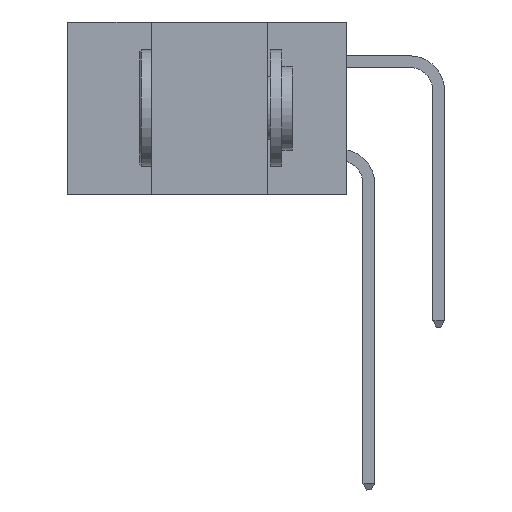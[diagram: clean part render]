
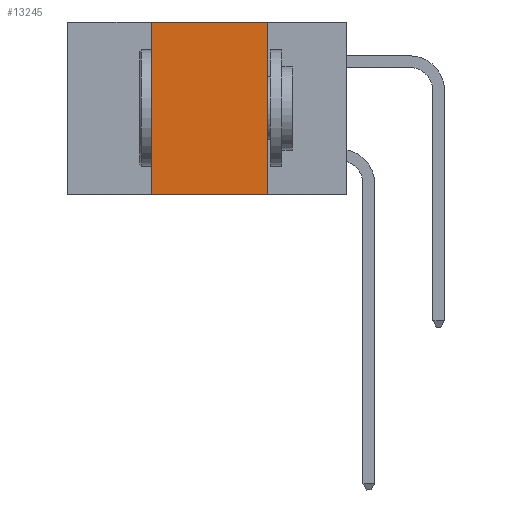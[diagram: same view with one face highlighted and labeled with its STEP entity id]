
A CAD part, left-side view. The second image highlights one B-rep face of the part: STEP entity #13245.
In plain terms, the highlighted planar face has unit normal (-1, 0, 0).
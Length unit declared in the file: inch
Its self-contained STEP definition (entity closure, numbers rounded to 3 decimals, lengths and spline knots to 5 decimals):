
#2314 = CARTESIAN_POINT ( 'NONE',  ( 0., 0.6, 0. ) ) ;
#2728 = VECTOR ( 'NONE', #20576, 39.37008 ) ;
#3229 = VERTEX_POINT ( 'NONE', #11223 ) ;
#3292 = EDGE_CURVE ( 'NONE', #20865, #9511, #11533, .T. ) ;
#3324 = EDGE_CURVE ( 'NONE', #19176, #20865, #10949, .T. ) ;
#3761 = CARTESIAN_POINT ( 'NONE',  ( 0., 0.42, 0. ) ) ;
#4230 = PLANE ( 'NONE',  #18257 ) ;
#5069 = DIRECTION ( 'NONE',  ( 0., 0., -1. ) ) ;
#7204 = VECTOR ( 'NONE', #10216, 39.37008 ) ;
#7755 = LINE ( 'NONE', #9397, #2728 ) ;
#7993 = DIRECTION ( 'NONE',  ( 1., 0., 0. ) ) ;
#9397 = CARTESIAN_POINT ( 'NONE',  ( 0., 0.6, -0.37 ) ) ;
#9511 = VERTEX_POINT ( 'NONE', #19887 ) ;
#9880 = CARTESIAN_POINT ( 'NONE',  ( 0., 0.42, 0. ) ) ;
#10057 = DIRECTION ( 'NONE',  ( 0., 0., 1. ) ) ;
#10216 = DIRECTION ( 'NONE',  ( 0., -1., 0. ) ) ;
#10287 = CARTESIAN_POINT ( 'NONE',  ( 0., 0.6, 0. ) ) ;
#10684 = ORIENTED_EDGE ( 'NONE', *, *, #3292, .F. ) ;
#10949 = LINE ( 'NONE', #9880, #20304 ) ;
#11223 = CARTESIAN_POINT ( 'NONE',  ( 0., 0.17, -0.37 ) ) ;
#11476 = LINE ( 'NONE', #19953, #15794 ) ;
#11533 = LINE ( 'NONE', #10287, #7204 ) ;
#12134 = ORIENTED_EDGE ( 'NONE', *, *, #22570, .F. ) ;
#13245 = ADVANCED_FACE ( 'NONE', ( #15724 ), #4230, .F. ) ;
#15724 = FACE_OUTER_BOUND ( 'NONE', #16061, .T. ) ;
#15794 = VECTOR ( 'NONE', #5069, 39.37008 ) ;
#16061 = EDGE_LOOP ( 'NONE', ( #12134, #10684, #22403, #19147 ) ) ;
#18257 = AXIS2_PLACEMENT_3D ( 'NONE', #2314, #7993, #21038 ) ;
#19147 = ORIENTED_EDGE ( 'NONE', *, *, #22100, .T. ) ;
#19176 = VERTEX_POINT ( 'NONE', #22909 ) ;
#19887 = CARTESIAN_POINT ( 'NONE',  ( 0., 0.17, 0. ) ) ;
#19953 = CARTESIAN_POINT ( 'NONE',  ( 0., 0.17, 0. ) ) ;
#20304 = VECTOR ( 'NONE', #10057, 39.37008 ) ;
#20576 = DIRECTION ( 'NONE',  ( 0., -1., 0. ) ) ;
#20865 = VERTEX_POINT ( 'NONE', #3761 ) ;
#21038 = DIRECTION ( 'NONE',  ( 0., 0., -1. ) ) ;
#22100 = EDGE_CURVE ( 'NONE', #19176, #3229, #7755, .T. ) ;
#22403 = ORIENTED_EDGE ( 'NONE', *, *, #3324, .F. ) ;
#22570 = EDGE_CURVE ( 'NONE', #9511, #3229, #11476, .T. ) ;
#22909 = CARTESIAN_POINT ( 'NONE',  ( 0., 0.42, -0.37 ) ) ;
